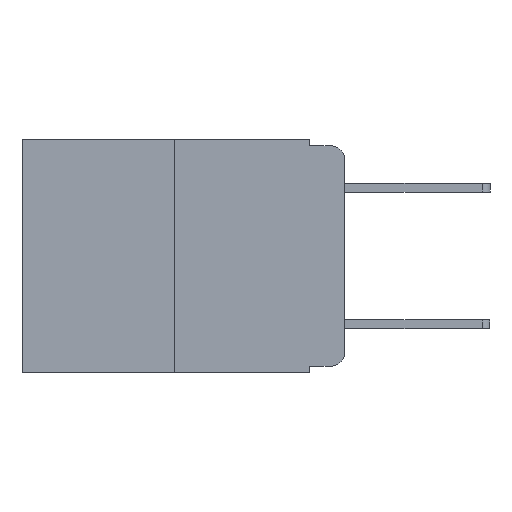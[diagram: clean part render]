
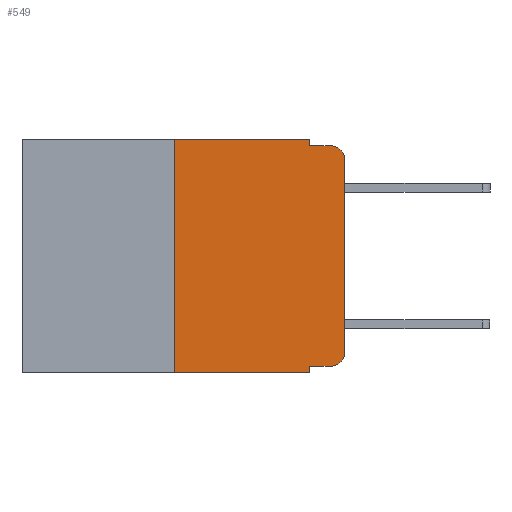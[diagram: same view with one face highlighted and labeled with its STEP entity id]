
A CAD part, left-side view. The second image highlights one B-rep face of the part: STEP entity #549.
In plain terms, the highlighted planar face has unit normal (-1, 0, 0).
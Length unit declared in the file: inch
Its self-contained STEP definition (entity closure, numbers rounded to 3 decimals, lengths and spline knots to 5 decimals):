
#311 = CIRCLE ( 'NONE', #9628, 0.02 ) ;
#448 = VERTEX_POINT ( 'NONE', #11531 ) ;
#501 = CARTESIAN_POINT ( 'NONE',  ( 0., 0.051, 0. ) ) ;
#549 = ADVANCED_FACE ( 'NONE', ( #8861 ), #1311, .F. ) ;
#626 = VERTEX_POINT ( 'NONE', #16418 ) ;
#1089 = DIRECTION ( 'NONE',  ( 0., -1., 0. ) ) ;
#1136 = CARTESIAN_POINT ( 'NONE',  ( 0., 0.051, 0. ) ) ;
#1311 = PLANE ( 'NONE',  #13055 ) ;
#1578 = DIRECTION ( 'NONE',  ( 0., 0., -1. ) ) ;
#1950 = DIRECTION ( 'NONE',  ( 1., 0., 0. ) ) ;
#2145 = EDGE_CURVE ( 'NONE', #5173, #8535, #7615, .T. ) ;
#2425 = ORIENTED_EDGE ( 'NONE', *, *, #11326, .F. ) ;
#2629 = EDGE_CURVE ( 'NONE', #3258, #4940, #15817, .T. ) ;
#2738 = VECTOR ( 'NONE', #17688, 39.37008 ) ;
#2925 = VERTEX_POINT ( 'NONE', #6525 ) ;
#2971 = DIRECTION ( 'NONE',  ( -1., 0., 0. ) ) ;
#3026 = ORIENTED_EDGE ( 'NONE', *, *, #15135, .F. ) ;
#3243 = ORIENTED_EDGE ( 'NONE', *, *, #2629, .F. ) ;
#3258 = VERTEX_POINT ( 'NONE', #4616 ) ;
#3275 = ORIENTED_EDGE ( 'NONE', *, *, #15986, .T. ) ;
#3359 = LINE ( 'NONE', #8067, #6968 ) ;
#3407 = CARTESIAN_POINT ( 'NONE',  ( 0., 0.051, 0. ) ) ;
#3521 = VECTOR ( 'NONE', #1089, 39.37008 ) ;
#3739 = ORIENTED_EDGE ( 'NONE', *, *, #13666, .T. ) ;
#4616 = CARTESIAN_POINT ( 'NONE',  ( 0., 0.051, -0.01 ) ) ;
#4849 = ORIENTED_EDGE ( 'NONE', *, *, #19040, .T. ) ;
#4940 = VERTEX_POINT ( 'NONE', #15862 ) ;
#5004 = ORIENTED_EDGE ( 'NONE', *, *, #12916, .T. ) ;
#5043 = VECTOR ( 'NONE', #10889, 39.37008 ) ;
#5068 = VERTEX_POINT ( 'NONE', #1136 ) ;
#5107 = ORIENTED_EDGE ( 'NONE', *, *, #12540, .F. ) ;
#5173 = VERTEX_POINT ( 'NONE', #7627 ) ;
#5269 = ORIENTED_EDGE ( 'NONE', *, *, #13992, .T. ) ;
#5288 = ORIENTED_EDGE ( 'NONE', *, *, #2145, .F. ) ;
#5623 = VECTOR ( 'NONE', #15566, 39.37008 ) ;
#6196 = CARTESIAN_POINT ( 'NONE',  ( 0., 0.25, 0. ) ) ;
#6525 = CARTESIAN_POINT ( 'NONE',  ( 0., 0., -0.03 ) ) ;
#6528 = CARTESIAN_POINT ( 'NONE',  ( 0., 0.02, -0.03 ) ) ;
#6917 = DIRECTION ( 'NONE',  ( 0., 0., 1. ) ) ;
#6933 = CARTESIAN_POINT ( 'NONE',  ( 0., 0.25, 0. ) ) ;
#6968 = VECTOR ( 'NONE', #16746, 39.37008 ) ;
#7615 = LINE ( 'NONE', #6933, #11480 ) ;
#7627 = CARTESIAN_POINT ( 'NONE',  ( 0., 0.25, -0.343 ) ) ;
#7636 = DIRECTION ( 'NONE',  ( 0., -1., 0. ) ) ;
#7723 = VERTEX_POINT ( 'NONE', #19081 ) ;
#7786 = AXIS2_PLACEMENT_3D ( 'NONE', #11935, #2971, #13424 ) ;
#8030 = DIRECTION ( 'NONE',  ( 0., 0., -1. ) ) ;
#8067 = CARTESIAN_POINT ( 'NONE',  ( 0., 0.473, -0.343 ) ) ;
#8535 = VERTEX_POINT ( 'NONE', #6196 ) ;
#8861 = FACE_OUTER_BOUND ( 'NONE', #18764, .T. ) ;
#9314 = CARTESIAN_POINT ( 'NONE',  ( 0., 0.473, 0. ) ) ;
#9528 = VERTEX_POINT ( 'NONE', #14277 ) ;
#9558 = VECTOR ( 'NONE', #11508, 39.37008 ) ;
#9628 = AXIS2_PLACEMENT_3D ( 'NONE', #6528, #16707, #8030 ) ;
#10338 = LINE ( 'NONE', #16255, #2738 ) ;
#10453 = LINE ( 'NONE', #3407, #5043 ) ;
#10889 = DIRECTION ( 'NONE',  ( 0., 0., -1. ) ) ;
#10932 = LINE ( 'NONE', #16349, #15255 ) ;
#11326 = EDGE_CURVE ( 'NONE', #8535, #5068, #10338, .T. ) ;
#11480 = VECTOR ( 'NONE', #6917, 39.37008 ) ;
#11508 = DIRECTION ( 'NONE',  ( 0., 0., 1. ) ) ;
#11531 = CARTESIAN_POINT ( 'NONE',  ( 0., 0., -0.313 ) ) ;
#11935 = CARTESIAN_POINT ( 'NONE',  ( 0., 0.02, -0.313 ) ) ;
#12540 = EDGE_CURVE ( 'NONE', #7723, #626, #13885, .T. ) ;
#12916 = EDGE_CURVE ( 'NONE', #7723, #9528, #10932, .T. ) ;
#13055 = AXIS2_PLACEMENT_3D ( 'NONE', #9314, #1950, #1578 ) ;
#13123 = CARTESIAN_POINT ( 'NONE',  ( 0., 0.051, -0.01 ) ) ;
#13424 = DIRECTION ( 'NONE',  ( 0., 0., -1. ) ) ;
#13666 = EDGE_CURVE ( 'NONE', #448, #2925, #13839, .T. ) ;
#13839 = LINE ( 'NONE', #18681, #9558 ) ;
#13885 = LINE ( 'NONE', #501, #5623 ) ;
#13992 = EDGE_CURVE ( 'NONE', #5173, #626, #3359, .T. ) ;
#14277 = CARTESIAN_POINT ( 'NONE',  ( 0., 0.02, -0.333 ) ) ;
#15135 = EDGE_CURVE ( 'NONE', #5068, #3258, #10453, .T. ) ;
#15255 = VECTOR ( 'NONE', #7636, 39.37008 ) ;
#15381 = CIRCLE ( 'NONE', #7786, 0.02 ) ;
#15566 = DIRECTION ( 'NONE',  ( 0., 0., -1. ) ) ;
#15817 = LINE ( 'NONE', #13123, #3521 ) ;
#15862 = CARTESIAN_POINT ( 'NONE',  ( 0., 0.02, -0.01 ) ) ;
#15986 = EDGE_CURVE ( 'NONE', #2925, #4940, #311, .T. ) ;
#16255 = CARTESIAN_POINT ( 'NONE',  ( 0., 0.473, 0. ) ) ;
#16349 = CARTESIAN_POINT ( 'NONE',  ( 0., 0.051, -0.333 ) ) ;
#16418 = CARTESIAN_POINT ( 'NONE',  ( 0., 0.051, -0.343 ) ) ;
#16707 = DIRECTION ( 'NONE',  ( -1., 0., 0. ) ) ;
#16746 = DIRECTION ( 'NONE',  ( 0., -1., 0. ) ) ;
#17688 = DIRECTION ( 'NONE',  ( 0., -1., 0. ) ) ;
#18681 = CARTESIAN_POINT ( 'NONE',  ( 0., 0., 0. ) ) ;
#18764 = EDGE_LOOP ( 'NONE', ( #3739, #3275, #3243, #3026, #2425, #5288, #5269, #5107, #5004, #4849 ) ) ;
#19040 = EDGE_CURVE ( 'NONE', #9528, #448, #15381, .T. ) ;
#19081 = CARTESIAN_POINT ( 'NONE',  ( 0., 0.051, -0.333 ) ) ;
